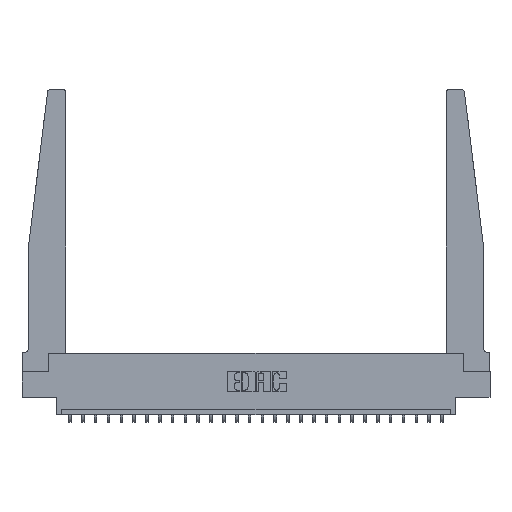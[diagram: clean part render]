
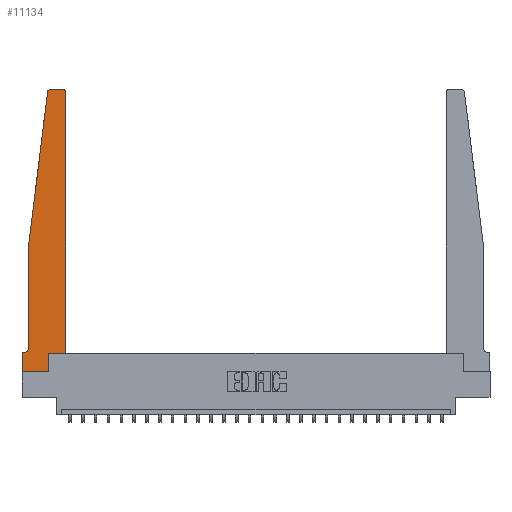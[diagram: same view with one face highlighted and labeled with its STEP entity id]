
A CAD part, top view. The second image highlights one B-rep face of the part: STEP entity #11134.
In plain terms, the highlighted planar face has unit normal (0, 0, 1).
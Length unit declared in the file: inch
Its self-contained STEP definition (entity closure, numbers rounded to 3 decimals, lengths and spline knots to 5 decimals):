
#118 = CARTESIAN_POINT ( 'NONE',  ( 0., 0.1875, 0.37 ) ) ;
#357 = EDGE_CURVE ( 'NONE', #9896, #2384, #21433, .T. ) ;
#653 = PLANE ( 'NONE',  #6899 ) ;
#715 = DIRECTION ( 'NONE',  ( -1., 0., 0. ) ) ;
#1028 = EDGE_CURVE ( 'NONE', #2384, #22373, #7386, .T. ) ;
#1350 = EDGE_CURVE ( 'NONE', #13802, #17933, #9830, .T. ) ;
#1451 = LINE ( 'NONE', #14360, #16443 ) ;
#1834 = DIRECTION ( 'NONE',  ( 0., -1., 0. ) ) ;
#2237 = LINE ( 'NONE', #18208, #22329 ) ;
#2384 = VERTEX_POINT ( 'NONE', #24549 ) ;
#2880 = DIRECTION ( 'NONE',  ( 0., 1., 0. ) ) ;
#3488 = CARTESIAN_POINT ( 'NONE',  ( 0., 0., 0.37 ) ) ;
#4027 = VECTOR ( 'NONE', #8535, 39.37008 ) ;
#4187 = AXIS2_PLACEMENT_3D ( 'NONE', #8596, #22192, #10543 ) ;
#4543 = LINE ( 'NONE', #4744, #24056 ) ;
#4731 = LINE ( 'NONE', #3488, #15120 ) ;
#4744 = CARTESIAN_POINT ( 'NONE',  ( 0.2605, 0.18, 0.37 ) ) ;
#4857 = DIRECTION ( 'NONE',  ( 1., 0., 0. ) ) ;
#5013 = CARTESIAN_POINT ( 'NONE',  ( 0.015, 0.1875, 0.37 ) ) ;
#5169 = CIRCLE ( 'NONE', #14910, 0.05 ) ;
#5686 = ORIENTED_EDGE ( 'NONE', *, *, #14557, .T. ) ;
#6088 = CARTESIAN_POINT ( 'NONE',  ( 0.015, 0.2375, 0.37 ) ) ;
#6090 = AXIS2_PLACEMENT_3D ( 'NONE', #13733, #14017, #13844 ) ;
#6590 = DIRECTION ( 'NONE',  ( 1., 0., 0. ) ) ;
#6787 = VECTOR ( 'NONE', #11274, 39.37008 ) ;
#6899 = AXIS2_PLACEMENT_3D ( 'NONE', #14375, #18298, #6590 ) ;
#7220 = ORIENTED_EDGE ( 'NONE', *, *, #20741, .T. ) ;
#7386 = LINE ( 'NONE', #16876, #6787 ) ;
#7632 = VERTEX_POINT ( 'NONE', #7989 ) ;
#7970 = CIRCLE ( 'NONE', #4187, 0.03 ) ;
#7974 = CARTESIAN_POINT ( 'NONE',  ( 0.425, 0.18, 0.37 ) ) ;
#7989 = CARTESIAN_POINT ( 'NONE',  ( 0.395, 2.75, 0.37 ) ) ;
#8060 = DIRECTION ( 'NONE',  ( -1., 0., 0. ) ) ;
#8188 = VERTEX_POINT ( 'NONE', #9572 ) ;
#8190 = EDGE_CURVE ( 'NONE', #22373, #18512, #8670, .T. ) ;
#8295 = VERTEX_POINT ( 'NONE', #118 ) ;
#8468 = CARTESIAN_POINT ( 'NONE',  ( 0.27653, 2.75, 0.37 ) ) ;
#8535 = DIRECTION ( 'NONE',  ( 1., 0., 0. ) ) ;
#8596 = CARTESIAN_POINT ( 'NONE',  ( 0.395, 2.72, 0.37 ) ) ;
#8670 = LINE ( 'NONE', #25136, #13218 ) ;
#8959 = EDGE_CURVE ( 'NONE', #7632, #9896, #11655, .T. ) ;
#9069 = ORIENTED_EDGE ( 'NONE', *, *, #357, .T. ) ;
#9572 = CARTESIAN_POINT ( 'NONE',  ( 0.2605, 0.18, 0.37 ) ) ;
#9830 = LINE ( 'NONE', #12438, #4027 ) ;
#9896 = VERTEX_POINT ( 'NONE', #8468 ) ;
#10543 = DIRECTION ( 'NONE',  ( 1., 0., 0. ) ) ;
#10973 = VERTEX_POINT ( 'NONE', #7974 ) ;
#10978 = EDGE_CURVE ( 'NONE', #18512, #16438, #5169, .T. ) ;
#11091 = CARTESIAN_POINT ( 'NONE',  ( 0.425, 2.72, 0.37 ) ) ;
#11134 = ADVANCED_FACE ( 'NONE', ( #21002 ), #653, .T. ) ;
#11162 = ORIENTED_EDGE ( 'NONE', *, *, #12508, .T. ) ;
#11186 = ORIENTED_EDGE ( 'NONE', *, *, #19256, .T. ) ;
#11191 = ORIENTED_EDGE ( 'NONE', *, *, #8959, .T. ) ;
#11274 = DIRECTION ( 'NONE',  ( -0.122, -0.992, 0. ) ) ;
#11655 = LINE ( 'NONE', #24027, #17484 ) ;
#12314 = CARTESIAN_POINT ( 'NONE',  ( 0., 0., 0.37 ) ) ;
#12339 = DIRECTION ( 'NONE',  ( -1., 0., 0. ) ) ;
#12438 = CARTESIAN_POINT ( 'NONE',  ( 0., 0., 0.37 ) ) ;
#12508 = EDGE_CURVE ( 'NONE', #16438, #8295, #1451, .T. ) ;
#12897 = CARTESIAN_POINT ( 'NONE',  ( 0.065, 0.2375, 0.37 ) ) ;
#13218 = VECTOR ( 'NONE', #1834, 39.37008 ) ;
#13674 = EDGE_LOOP ( 'NONE', ( #11191, #9069, #22779, #20329, #14891, #11162, #11186, #24016, #14866, #5686, #7220, #16714 ) ) ;
#13733 = CARTESIAN_POINT ( 'NONE',  ( 0.27653, 2.72, 0.37 ) ) ;
#13802 = VERTEX_POINT ( 'NONE', #12314 ) ;
#13844 = DIRECTION ( 'NONE',  ( 1., 0., 0. ) ) ;
#14017 = DIRECTION ( 'NONE',  ( 0., 0., 1. ) ) ;
#14360 = CARTESIAN_POINT ( 'NONE',  ( 0.065, 0.1875, 0.37 ) ) ;
#14375 = CARTESIAN_POINT ( 'NONE',  ( 0., 0.1875, 0.37 ) ) ;
#14413 = VECTOR ( 'NONE', #4857, 39.37008 ) ;
#14557 = EDGE_CURVE ( 'NONE', #8188, #10973, #19581, .T. ) ;
#14866 = ORIENTED_EDGE ( 'NONE', *, *, #24650, .T. ) ;
#14891 = ORIENTED_EDGE ( 'NONE', *, *, #10978, .T. ) ;
#14910 = AXIS2_PLACEMENT_3D ( 'NONE', #6088, #19734, #8060 ) ;
#15097 = EDGE_CURVE ( 'NONE', #21427, #7632, #7970, .T. ) ;
#15120 = VECTOR ( 'NONE', #19090, 39.37008 ) ;
#15781 = CARTESIAN_POINT ( 'NONE',  ( 0.065, 1.25, 0.37 ) ) ;
#16438 = VERTEX_POINT ( 'NONE', #5013 ) ;
#16443 = VECTOR ( 'NONE', #715, 39.37008 ) ;
#16714 = ORIENTED_EDGE ( 'NONE', *, *, #15097, .T. ) ;
#16876 = CARTESIAN_POINT ( 'NONE',  ( 0.065, 1.25, 0.37 ) ) ;
#17484 = VECTOR ( 'NONE', #12339, 39.37008 ) ;
#17933 = VERTEX_POINT ( 'NONE', #25036 ) ;
#18208 = CARTESIAN_POINT ( 'NONE',  ( 0.425, 0.18, 0.37 ) ) ;
#18298 = DIRECTION ( 'NONE',  ( 0., 0., 1. ) ) ;
#18512 = VERTEX_POINT ( 'NONE', #12897 ) ;
#19090 = DIRECTION ( 'NONE',  ( 0., -1., 0. ) ) ;
#19256 = EDGE_CURVE ( 'NONE', #8295, #13802, #4731, .T. ) ;
#19581 = LINE ( 'NONE', #24212, #14413 ) ;
#19734 = DIRECTION ( 'NONE',  ( 0., 0., -1. ) ) ;
#20329 = ORIENTED_EDGE ( 'NONE', *, *, #8190, .T. ) ;
#20741 = EDGE_CURVE ( 'NONE', #10973, #21427, #2237, .T. ) ;
#21002 = FACE_OUTER_BOUND ( 'NONE', #13674, .T. ) ;
#21427 = VERTEX_POINT ( 'NONE', #11091 ) ;
#21433 = CIRCLE ( 'NONE', #6090, 0.03 ) ;
#22070 = DIRECTION ( 'NONE',  ( 0., 1., 0. ) ) ;
#22192 = DIRECTION ( 'NONE',  ( 0., 0., 1. ) ) ;
#22329 = VECTOR ( 'NONE', #22070, 39.37008 ) ;
#22373 = VERTEX_POINT ( 'NONE', #15781 ) ;
#22779 = ORIENTED_EDGE ( 'NONE', *, *, #1028, .T. ) ;
#24016 = ORIENTED_EDGE ( 'NONE', *, *, #1350, .T. ) ;
#24027 = CARTESIAN_POINT ( 'NONE',  ( 0.25, 2.75, 0.37 ) ) ;
#24056 = VECTOR ( 'NONE', #2880, 39.37008 ) ;
#24212 = CARTESIAN_POINT ( 'NONE',  ( 0.425, 0.18, 0.37 ) ) ;
#24549 = CARTESIAN_POINT ( 'NONE',  ( 0.24675, 2.72367, 0.37 ) ) ;
#24650 = EDGE_CURVE ( 'NONE', #17933, #8188, #4543, .T. ) ;
#25036 = CARTESIAN_POINT ( 'NONE',  ( 0.2605, 0., 0.37 ) ) ;
#25136 = CARTESIAN_POINT ( 'NONE',  ( 0.065, 1.25, 0.37 ) ) ;
